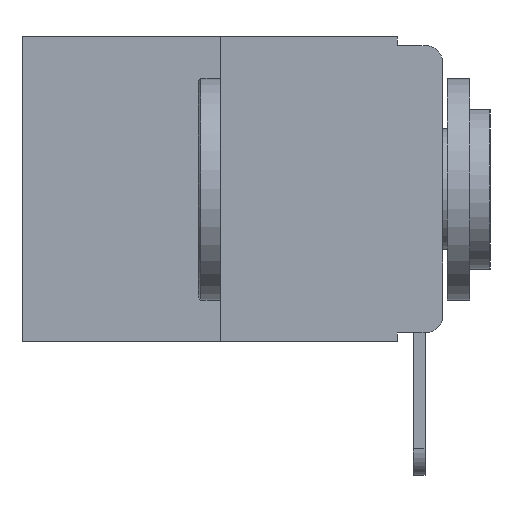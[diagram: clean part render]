
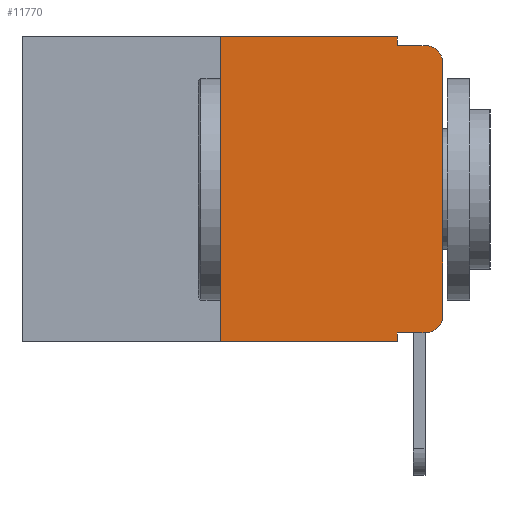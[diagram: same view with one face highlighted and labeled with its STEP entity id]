
A CAD part, left-side view. The second image highlights one B-rep face of the part: STEP entity #11770.
In plain terms, the highlighted planar face has unit normal (-1, 0, 0).
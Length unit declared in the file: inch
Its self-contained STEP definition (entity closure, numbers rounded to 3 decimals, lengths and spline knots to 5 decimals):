
#236 = DIRECTION ( 'NONE',  ( 1., 0., 0. ) ) ;
#252 = VERTEX_POINT ( 'NONE', #4819 ) ;
#637 = VECTOR ( 'NONE', #1389, 39.37008 ) ;
#737 = LINE ( 'NONE', #4971, #2521 ) ;
#937 = LINE ( 'NONE', #4065, #13590 ) ;
#1076 = VERTEX_POINT ( 'NONE', #9240 ) ;
#1146 = DIRECTION ( 'NONE',  ( 0., 0., 1. ) ) ;
#1273 = CARTESIAN_POINT ( 'NONE',  ( 0., 0.473, 0. ) ) ;
#1326 = VERTEX_POINT ( 'NONE', #10592 ) ;
#1389 = DIRECTION ( 'NONE',  ( 0., -1., 0. ) ) ;
#1617 = CARTESIAN_POINT ( 'NONE',  ( 0., 0.02, -0.03 ) ) ;
#1666 = EDGE_CURVE ( 'NONE', #9501, #5352, #937, .T. ) ;
#2070 = ORIENTED_EDGE ( 'NONE', *, *, #9409, .T. ) ;
#2425 = VERTEX_POINT ( 'NONE', #4733 ) ;
#2505 = DIRECTION ( 'NONE',  ( 0., -1., 0. ) ) ;
#2521 = VECTOR ( 'NONE', #9230, 39.37008 ) ;
#2538 = EDGE_LOOP ( 'NONE', ( #11225, #2070, #3742, #10867, #8048, #12474, #5538, #11416, #12762, #7401 ) ) ;
#2858 = EDGE_CURVE ( 'NONE', #2425, #4934, #13423, .T. ) ;
#2917 = CARTESIAN_POINT ( 'NONE',  ( 0., 0.02, -0.333 ) ) ;
#2990 = CARTESIAN_POINT ( 'NONE',  ( 0., 0.25, 0. ) ) ;
#3077 = LINE ( 'NONE', #6416, #13331 ) ;
#3742 = ORIENTED_EDGE ( 'NONE', *, *, #7463, .F. ) ;
#4065 = CARTESIAN_POINT ( 'NONE',  ( 0., 0.25, 0. ) ) ;
#4207 = CARTESIAN_POINT ( 'NONE',  ( 0., 0.051, -0.333 ) ) ;
#4477 = FACE_OUTER_BOUND ( 'NONE', #2538, .T. ) ;
#4728 = CARTESIAN_POINT ( 'NONE',  ( 0., 0.02, -0.01 ) ) ;
#4733 = CARTESIAN_POINT ( 'NONE',  ( 0., 0., -0.313 ) ) ;
#4808 = DIRECTION ( 'NONE',  ( -1., 0., 0. ) ) ;
#4819 = CARTESIAN_POINT ( 'NONE',  ( 0., 0.051, 0. ) ) ;
#4910 = EDGE_CURVE ( 'NONE', #9501, #1326, #11406, .T. ) ;
#4934 = VERTEX_POINT ( 'NONE', #13724 ) ;
#4937 = CIRCLE ( 'NONE', #13672, 0.02 ) ;
#4949 = CARTESIAN_POINT ( 'NONE',  ( 0., 0.473, -0.343 ) ) ;
#4971 = CARTESIAN_POINT ( 'NONE',  ( 0., 0.051, -0.01 ) ) ;
#5352 = VERTEX_POINT ( 'NONE', #2990 ) ;
#5512 = EDGE_CURVE ( 'NONE', #13462, #1326, #9473, .T. ) ;
#5538 = ORIENTED_EDGE ( 'NONE', *, *, #4910, .T. ) ;
#5559 = VECTOR ( 'NONE', #11616, 39.37008 ) ;
#5567 = LINE ( 'NONE', #10962, #637 ) ;
#5934 = DIRECTION ( 'NONE',  ( 0., 0., -1. ) ) ;
#6416 = CARTESIAN_POINT ( 'NONE',  ( 0., 0.051, 0. ) ) ;
#6565 = DIRECTION ( 'NONE',  ( 0., 0., -1. ) ) ;
#6665 = LINE ( 'NONE', #7638, #11091 ) ;
#7401 = ORIENTED_EDGE ( 'NONE', *, *, #7907, .T. ) ;
#7463 = EDGE_CURVE ( 'NONE', #1076, #11030, #737, .T. ) ;
#7503 = DIRECTION ( 'NONE',  ( 0., 0., -1. ) ) ;
#7604 = DIRECTION ( 'NONE',  ( 0., 0., -1. ) ) ;
#7638 = CARTESIAN_POINT ( 'NONE',  ( 0., 0.051, -0.333 ) ) ;
#7667 = DIRECTION ( 'NONE',  ( -1., 0., 0. ) ) ;
#7907 = EDGE_CURVE ( 'NONE', #11232, #2425, #4937, .T. ) ;
#8006 = VECTOR ( 'NONE', #7503, 39.37008 ) ;
#8048 = ORIENTED_EDGE ( 'NONE', *, *, #11630, .F. ) ;
#9230 = DIRECTION ( 'NONE',  ( 0., -1., 0. ) ) ;
#9240 = CARTESIAN_POINT ( 'NONE',  ( 0., 0.051, -0.01 ) ) ;
#9293 = EDGE_CURVE ( 'NONE', #252, #1076, #3077, .T. ) ;
#9409 = EDGE_CURVE ( 'NONE', #4934, #11030, #10169, .T. ) ;
#9473 = LINE ( 'NONE', #9543, #8006 ) ;
#9501 = VERTEX_POINT ( 'NONE', #11118 ) ;
#9543 = CARTESIAN_POINT ( 'NONE',  ( 0., 0.051, 0. ) ) ;
#9763 = EDGE_CURVE ( 'NONE', #13462, #11232, #6665, .T. ) ;
#10046 = DIRECTION ( 'NONE',  ( 0., 0., 1. ) ) ;
#10116 = CARTESIAN_POINT ( 'NONE',  ( 0., 0., 0. ) ) ;
#10169 = CIRCLE ( 'NONE', #12867, 0.02 ) ;
#10592 = CARTESIAN_POINT ( 'NONE',  ( 0., 0.051, -0.343 ) ) ;
#10867 = ORIENTED_EDGE ( 'NONE', *, *, #9293, .F. ) ;
#10962 = CARTESIAN_POINT ( 'NONE',  ( 0., 0.473, 0. ) ) ;
#11030 = VERTEX_POINT ( 'NONE', #4728 ) ;
#11091 = VECTOR ( 'NONE', #2505, 39.37008 ) ;
#11118 = CARTESIAN_POINT ( 'NONE',  ( 0., 0.25, -0.343 ) ) ;
#11133 = CARTESIAN_POINT ( 'NONE',  ( 0., 0.02, -0.313 ) ) ;
#11225 = ORIENTED_EDGE ( 'NONE', *, *, #2858, .T. ) ;
#11232 = VERTEX_POINT ( 'NONE', #2917 ) ;
#11406 = LINE ( 'NONE', #4949, #5559 ) ;
#11416 = ORIENTED_EDGE ( 'NONE', *, *, #5512, .F. ) ;
#11616 = DIRECTION ( 'NONE',  ( 0., -1., 0. ) ) ;
#11630 = EDGE_CURVE ( 'NONE', #5352, #252, #5567, .T. ) ;
#11770 = ADVANCED_FACE ( 'NONE', ( #4477 ), #11908, .F. ) ;
#11812 = AXIS2_PLACEMENT_3D ( 'NONE', #1273, #236, #6565 ) ;
#11908 = PLANE ( 'NONE',  #11812 ) ;
#12474 = ORIENTED_EDGE ( 'NONE', *, *, #1666, .F. ) ;
#12762 = ORIENTED_EDGE ( 'NONE', *, *, #9763, .T. ) ;
#12867 = AXIS2_PLACEMENT_3D ( 'NONE', #1617, #7667, #13300 ) ;
#13300 = DIRECTION ( 'NONE',  ( 0., 0., -1. ) ) ;
#13331 = VECTOR ( 'NONE', #7604, 39.37008 ) ;
#13423 = LINE ( 'NONE', #10116, #13594 ) ;
#13462 = VERTEX_POINT ( 'NONE', #4207 ) ;
#13590 = VECTOR ( 'NONE', #1146, 39.37008 ) ;
#13594 = VECTOR ( 'NONE', #10046, 39.37008 ) ;
#13672 = AXIS2_PLACEMENT_3D ( 'NONE', #11133, #4808, #5934 ) ;
#13724 = CARTESIAN_POINT ( 'NONE',  ( 0., 0., -0.03 ) ) ;
